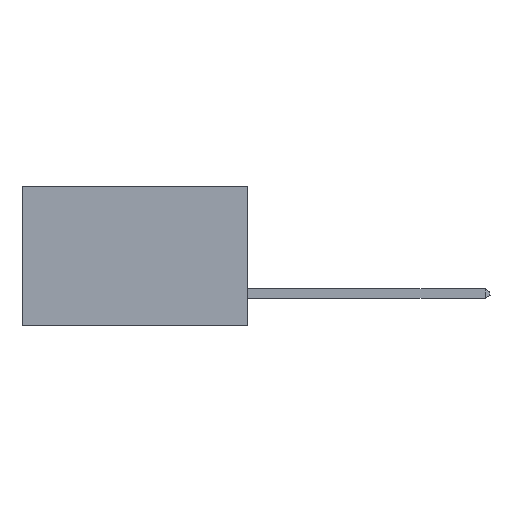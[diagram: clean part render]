
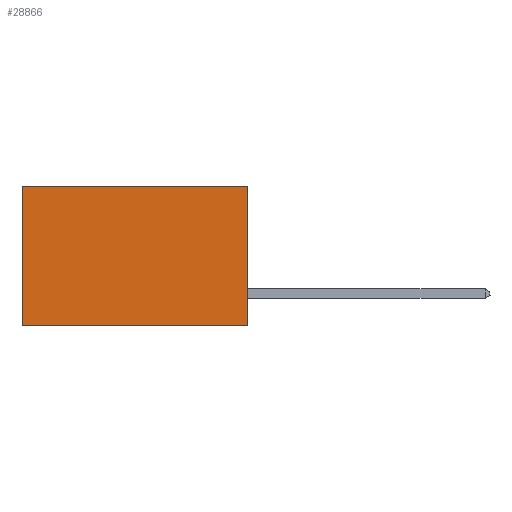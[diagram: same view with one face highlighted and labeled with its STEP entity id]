
A CAD part, left-side view. The second image highlights one B-rep face of the part: STEP entity #28866.
In plain terms, the highlighted planar face has unit normal (-1, 0, 0).
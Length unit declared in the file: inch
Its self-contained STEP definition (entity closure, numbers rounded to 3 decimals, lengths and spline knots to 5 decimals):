
#258 = VERTEX_POINT ( 'NONE', #29022 ) ;
#1985 = CARTESIAN_POINT ( 'NONE',  ( 0.298, 0., 0. ) ) ;
#2025 = EDGE_LOOP ( 'NONE', ( #18523, #15965, #3260, #15056 ) ) ;
#2060 = EDGE_CURVE ( 'NONE', #7946, #258, #30818, .T. ) ;
#2381 = CARTESIAN_POINT ( 'NONE',  ( 0.298, 0., 0. ) ) ;
#3260 = ORIENTED_EDGE ( 'NONE', *, *, #2060, .F. ) ;
#3638 = CARTESIAN_POINT ( 'NONE',  ( 0.298, 0.6, 0. ) ) ;
#4789 = DIRECTION ( 'NONE',  ( 0., 0., -1. ) ) ;
#5170 = VECTOR ( 'NONE', #30321, 39.37008 ) ;
#7946 = VERTEX_POINT ( 'NONE', #23129 ) ;
#10998 = VERTEX_POINT ( 'NONE', #15878 ) ;
#11247 = FACE_OUTER_BOUND ( 'NONE', #2025, .T. ) ;
#11452 = VECTOR ( 'NONE', #25643, 39.37008 ) ;
#11734 = DIRECTION ( 'NONE',  ( 0., 1., 0. ) ) ;
#12314 = LINE ( 'NONE', #23026, #5170 ) ;
#13391 = DIRECTION ( 'NONE',  ( 0., 0., -1. ) ) ;
#13754 = VECTOR ( 'NONE', #11734, 39.37008 ) ;
#15056 = ORIENTED_EDGE ( 'NONE', *, *, #29537, .T. ) ;
#15315 = AXIS2_PLACEMENT_3D ( 'NONE', #2381, #19158, #4789 ) ;
#15878 = CARTESIAN_POINT ( 'NONE',  ( 0.298, 0.6, 0. ) ) ;
#15965 = ORIENTED_EDGE ( 'NONE', *, *, #29980, .F. ) ;
#16210 = CARTESIAN_POINT ( 'NONE',  ( 0.298, 0., -0.37 ) ) ;
#18523 = ORIENTED_EDGE ( 'NONE', *, *, #30882, .T. ) ;
#19158 = DIRECTION ( 'NONE',  ( 1., 0., 0. ) ) ;
#21685 = CARTESIAN_POINT ( 'NONE',  ( 0.298, 0.6, -0.37 ) ) ;
#22027 = PLANE ( 'NONE',  #15315 ) ;
#23026 = CARTESIAN_POINT ( 'NONE',  ( 0.298, 0., 0. ) ) ;
#23028 = VECTOR ( 'NONE', #13391, 39.37008 ) ;
#23129 = CARTESIAN_POINT ( 'NONE',  ( 0.298, 0., 0. ) ) ;
#24587 = LINE ( 'NONE', #16210, #13754 ) ;
#25643 = DIRECTION ( 'NONE',  ( 0., 0., -1. ) ) ;
#28866 = ADVANCED_FACE ( 'NONE', ( #11247 ), #22027, .F. ) ;
#29022 = CARTESIAN_POINT ( 'NONE',  ( 0.298, 0., -0.37 ) ) ;
#29206 = VERTEX_POINT ( 'NONE', #21685 ) ;
#29386 = LINE ( 'NONE', #3638, #23028 ) ;
#29537 = EDGE_CURVE ( 'NONE', #7946, #10998, #12314, .T. ) ;
#29980 = EDGE_CURVE ( 'NONE', #258, #29206, #24587, .T. ) ;
#30321 = DIRECTION ( 'NONE',  ( 0., 1., 0. ) ) ;
#30818 = LINE ( 'NONE', #1985, #11452 ) ;
#30882 = EDGE_CURVE ( 'NONE', #10998, #29206, #29386, .T. ) ;
